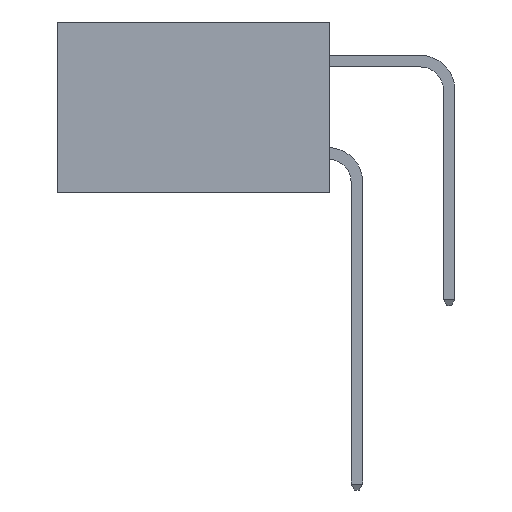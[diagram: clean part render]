
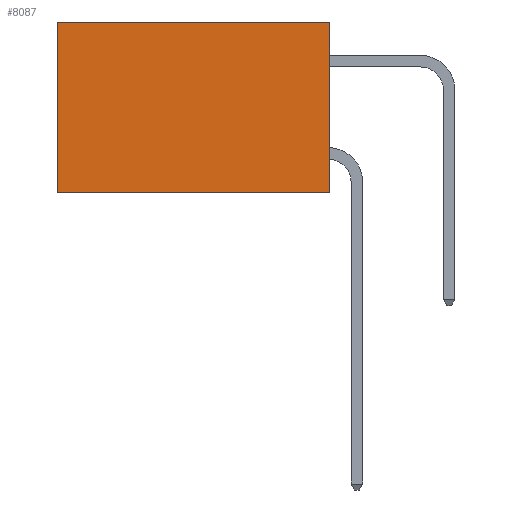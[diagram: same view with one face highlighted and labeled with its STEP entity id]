
A CAD part, left-side view. The second image highlights one B-rep face of the part: STEP entity #8087.
In plain terms, the highlighted planar face has unit normal (-1, 0, 0).
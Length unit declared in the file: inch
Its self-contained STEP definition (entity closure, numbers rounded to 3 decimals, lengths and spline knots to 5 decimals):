
#240 = VECTOR ( 'NONE', #8471, 39.37008 ) ;
#355 = DIRECTION ( 'NONE',  ( 0., 0., -1. ) ) ;
#892 = CARTESIAN_POINT ( 'NONE',  ( 0.277, 0., -0.37 ) ) ;
#986 = VERTEX_POINT ( 'NONE', #4127 ) ;
#1264 = DIRECTION ( 'NONE',  ( 0., 0., -1. ) ) ;
#1265 = CARTESIAN_POINT ( 'NONE',  ( 0.277, 0.59, -0.37 ) ) ;
#1500 = LINE ( 'NONE', #1265, #7487 ) ;
#1820 = EDGE_CURVE ( 'NONE', #5612, #2917, #5331, .T. ) ;
#1985 = VECTOR ( 'NONE', #4443, 39.37008 ) ;
#2049 = ORIENTED_EDGE ( 'NONE', *, *, #5828, .F. ) ;
#2663 = CARTESIAN_POINT ( 'NONE',  ( 0.277, 0., -0.37 ) ) ;
#2917 = VERTEX_POINT ( 'NONE', #5304 ) ;
#3273 = DIRECTION ( 'NONE',  ( 0., 1., 0. ) ) ;
#3294 = CARTESIAN_POINT ( 'NONE',  ( 0.277, 0., -0.37 ) ) ;
#3367 = EDGE_CURVE ( 'NONE', #3744, #986, #9270, .T. ) ;
#3611 = EDGE_CURVE ( 'NONE', #2917, #986, #1500, .T. ) ;
#3744 = VERTEX_POINT ( 'NONE', #892 ) ;
#3774 = CARTESIAN_POINT ( 'NONE',  ( 0.277, 0., 0. ) ) ;
#4030 = ORIENTED_EDGE ( 'NONE', *, *, #1820, .T. ) ;
#4127 = CARTESIAN_POINT ( 'NONE',  ( 0.277, 0.59, -0.37 ) ) ;
#4443 = DIRECTION ( 'NONE',  ( 0., 1., 0. ) ) ;
#4550 = ORIENTED_EDGE ( 'NONE', *, *, #3611, .T. ) ;
#4743 = ORIENTED_EDGE ( 'NONE', *, *, #3367, .F. ) ;
#4769 = DIRECTION ( 'NONE',  ( 1., 0., 0. ) ) ;
#5148 = FACE_OUTER_BOUND ( 'NONE', #6932, .T. ) ;
#5304 = CARTESIAN_POINT ( 'NONE',  ( 0.277, 0.59, 0. ) ) ;
#5331 = LINE ( 'NONE', #9198, #1985 ) ;
#5612 = VERTEX_POINT ( 'NONE', #3774 ) ;
#5828 = EDGE_CURVE ( 'NONE', #5612, #3744, #6309, .T. ) ;
#6090 = AXIS2_PLACEMENT_3D ( 'NONE', #2663, #4769, #355 ) ;
#6309 = LINE ( 'NONE', #8493, #240 ) ;
#6932 = EDGE_LOOP ( 'NONE', ( #4550, #4743, #2049, #4030 ) ) ;
#7392 = VECTOR ( 'NONE', #3273, 39.37008 ) ;
#7487 = VECTOR ( 'NONE', #1264, 39.37008 ) ;
#8087 = ADVANCED_FACE ( 'NONE', ( #5148 ), #8886, .F. ) ;
#8471 = DIRECTION ( 'NONE',  ( 0., 0., -1. ) ) ;
#8493 = CARTESIAN_POINT ( 'NONE',  ( 0.277, 0., -0.37 ) ) ;
#8886 = PLANE ( 'NONE',  #6090 ) ;
#9198 = CARTESIAN_POINT ( 'NONE',  ( 0.277, 0., 0. ) ) ;
#9270 = LINE ( 'NONE', #3294, #7392 ) ;
